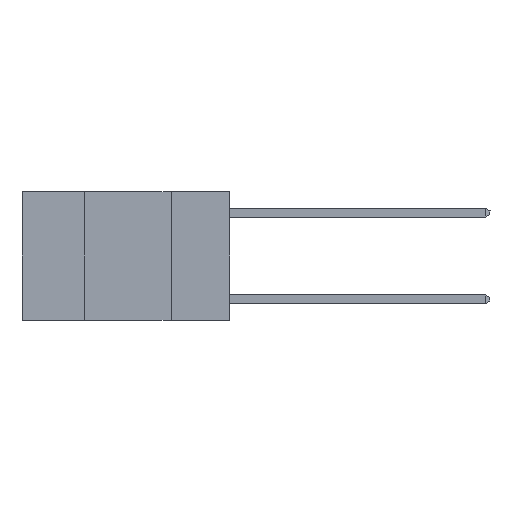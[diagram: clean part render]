
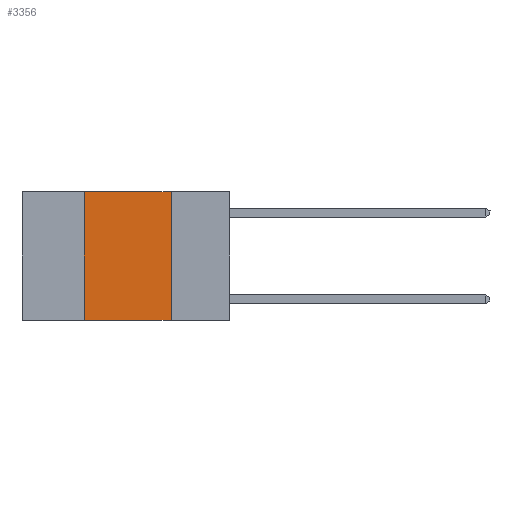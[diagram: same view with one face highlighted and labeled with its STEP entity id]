
A CAD part, left-side view. The second image highlights one B-rep face of the part: STEP entity #3356.
In plain terms, the highlighted planar face has unit normal (-1, 0, 0).
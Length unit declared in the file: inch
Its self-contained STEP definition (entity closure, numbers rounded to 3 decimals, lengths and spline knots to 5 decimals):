
#125 = CARTESIAN_POINT ( 'NONE',  ( 0., 0.6, -0.37 ) ) ;
#179 = DIRECTION ( 'NONE',  ( 1., 0., 0. ) ) ;
#221 = PLANE ( 'NONE',  #3199 ) ;
#284 = ORIENTED_EDGE ( 'NONE', *, *, #7367, .F. ) ;
#315 = CARTESIAN_POINT ( 'NONE',  ( 0., 0.17, -0.37 ) ) ;
#361 = EDGE_CURVE ( 'NONE', #3748, #6553, #2865, .T. ) ;
#474 = CARTESIAN_POINT ( 'NONE',  ( 0., 0.42, 0. ) ) ;
#497 = VERTEX_POINT ( 'NONE', #474 ) ;
#551 = ORIENTED_EDGE ( 'NONE', *, *, #5000, .F. ) ;
#800 = LINE ( 'NONE', #125, #1093 ) ;
#870 = DIRECTION ( 'NONE',  ( 0., 0., -1. ) ) ;
#1087 = VECTOR ( 'NONE', #3526, 39.37008 ) ;
#1093 = VECTOR ( 'NONE', #6933, 39.37008 ) ;
#1221 = CARTESIAN_POINT ( 'NONE',  ( 0., 0.42, -0.37 ) ) ;
#1555 = FACE_OUTER_BOUND ( 'NONE', #7958, .T. ) ;
#1882 = VECTOR ( 'NONE', #3969, 39.37008 ) ;
#2865 = LINE ( 'NONE', #4589, #1087 ) ;
#3199 = AXIS2_PLACEMENT_3D ( 'NONE', #4272, #179, #870 ) ;
#3243 = DIRECTION ( 'NONE',  ( 0., 0., 1. ) ) ;
#3356 = ADVANCED_FACE ( 'NONE', ( #1555 ), #221, .F. ) ;
#3526 = DIRECTION ( 'NONE',  ( 0., 0., -1. ) ) ;
#3748 = VERTEX_POINT ( 'NONE', #4938 ) ;
#3917 = ORIENTED_EDGE ( 'NONE', *, *, #361, .F. ) ;
#3969 = DIRECTION ( 'NONE',  ( 0., -1., 0. ) ) ;
#4272 = CARTESIAN_POINT ( 'NONE',  ( 0., 0.6, 0. ) ) ;
#4589 = CARTESIAN_POINT ( 'NONE',  ( 0., 0.17, 0. ) ) ;
#4938 = CARTESIAN_POINT ( 'NONE',  ( 0., 0.17, 0. ) ) ;
#5000 = EDGE_CURVE ( 'NONE', #5902, #497, #5398, .T. ) ;
#5017 = VECTOR ( 'NONE', #3243, 39.37008 ) ;
#5398 = LINE ( 'NONE', #7316, #5017 ) ;
#5654 = EDGE_CURVE ( 'NONE', #5902, #6553, #800, .T. ) ;
#5902 = VERTEX_POINT ( 'NONE', #1221 ) ;
#6126 = ORIENTED_EDGE ( 'NONE', *, *, #5654, .T. ) ;
#6553 = VERTEX_POINT ( 'NONE', #315 ) ;
#6933 = DIRECTION ( 'NONE',  ( 0., -1., 0. ) ) ;
#7316 = CARTESIAN_POINT ( 'NONE',  ( 0., 0.42, 0. ) ) ;
#7367 = EDGE_CURVE ( 'NONE', #497, #3748, #8715, .T. ) ;
#7377 = CARTESIAN_POINT ( 'NONE',  ( 0., 0.6, 0. ) ) ;
#7958 = EDGE_LOOP ( 'NONE', ( #3917, #284, #551, #6126 ) ) ;
#8715 = LINE ( 'NONE', #7377, #1882 ) ;
